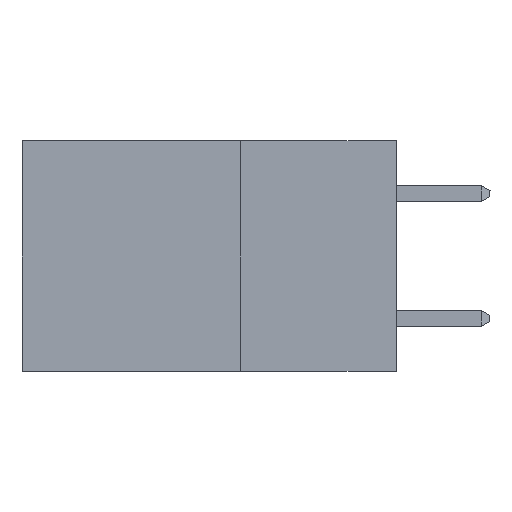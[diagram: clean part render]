
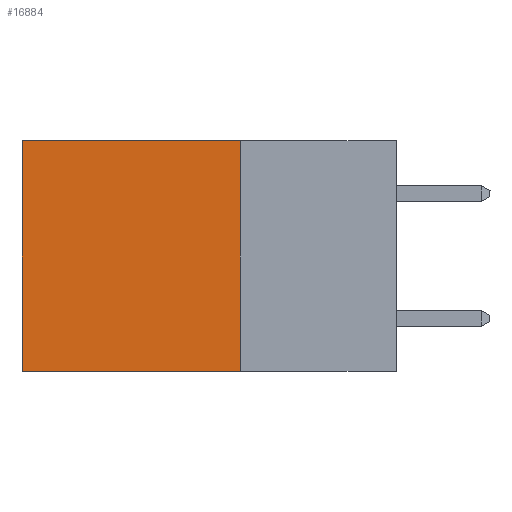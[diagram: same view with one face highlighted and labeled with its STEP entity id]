
A CAD part, left-side view. The second image highlights one B-rep face of the part: STEP entity #16884.
In plain terms, the highlighted planar face has unit normal (-1, 0, 0).
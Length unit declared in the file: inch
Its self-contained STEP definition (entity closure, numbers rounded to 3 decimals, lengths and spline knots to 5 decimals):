
#1252 = EDGE_CURVE ( 'NONE', #13404, #5144, #9243, .T. ) ;
#2403 = PLANE ( 'NONE',  #3668 ) ;
#2669 = ORIENTED_EDGE ( 'NONE', *, *, #17955, .T. ) ;
#3668 = AXIS2_PLACEMENT_3D ( 'NONE', #14720, #4499, #18843 ) ;
#4201 = CARTESIAN_POINT ( 'NONE',  ( 0.2615, 0.25, -0.37 ) ) ;
#4499 = DIRECTION ( 'NONE',  ( 1., 0., 0. ) ) ;
#4876 = EDGE_CURVE ( 'NONE', #19270, #9425, #12886, .T. ) ;
#5144 = VERTEX_POINT ( 'NONE', #4201 ) ;
#9243 = LINE ( 'NONE', #21538, #14675 ) ;
#9425 = VERTEX_POINT ( 'NONE', #18350 ) ;
#9893 = ORIENTED_EDGE ( 'NONE', *, *, #14242, .F. ) ;
#10083 = ORIENTED_EDGE ( 'NONE', *, *, #1252, .F. ) ;
#11781 = CARTESIAN_POINT ( 'NONE',  ( 0.2615, 0.6, -0.37 ) ) ;
#12010 = LINE ( 'NONE', #18688, #17463 ) ;
#12070 = DIRECTION ( 'NONE',  ( 0., 0., -1. ) ) ;
#12886 = LINE ( 'NONE', #11781, #22431 ) ;
#13404 = VERTEX_POINT ( 'NONE', #16873 ) ;
#14242 = EDGE_CURVE ( 'NONE', #5144, #9425, #12010, .T. ) ;
#14675 = VECTOR ( 'NONE', #21311, 39.37008 ) ;
#14682 = EDGE_LOOP ( 'NONE', ( #23050, #9893, #10083, #2669 ) ) ;
#14720 = CARTESIAN_POINT ( 'NONE',  ( 0.2615, 0.25, -0.37 ) ) ;
#15757 = VECTOR ( 'NONE', #22802, 39.37008 ) ;
#16873 = CARTESIAN_POINT ( 'NONE',  ( 0.2615, 0.25, 0. ) ) ;
#16884 = ADVANCED_FACE ( 'NONE', ( #23760 ), #2403, .F. ) ;
#17463 = VECTOR ( 'NONE', #24718, 39.37008 ) ;
#17955 = EDGE_CURVE ( 'NONE', #13404, #19270, #21166, .T. ) ;
#18350 = CARTESIAN_POINT ( 'NONE',  ( 0.2615, 0.6, -0.37 ) ) ;
#18688 = CARTESIAN_POINT ( 'NONE',  ( 0.2615, 0.25, -0.37 ) ) ;
#18843 = DIRECTION ( 'NONE',  ( 0., 0., -1. ) ) ;
#19270 = VERTEX_POINT ( 'NONE', #20891 ) ;
#20772 = CARTESIAN_POINT ( 'NONE',  ( 0.2615, 0.25, 0. ) ) ;
#20891 = CARTESIAN_POINT ( 'NONE',  ( 0.2615, 0.6, 0. ) ) ;
#21166 = LINE ( 'NONE', #20772, #15757 ) ;
#21311 = DIRECTION ( 'NONE',  ( 0., 0., -1. ) ) ;
#21538 = CARTESIAN_POINT ( 'NONE',  ( 0.2615, 0.25, -0.37 ) ) ;
#22431 = VECTOR ( 'NONE', #12070, 39.37008 ) ;
#22802 = DIRECTION ( 'NONE',  ( 0., 1., 0. ) ) ;
#23050 = ORIENTED_EDGE ( 'NONE', *, *, #4876, .T. ) ;
#23760 = FACE_OUTER_BOUND ( 'NONE', #14682, .T. ) ;
#24718 = DIRECTION ( 'NONE',  ( 0., 1., 0. ) ) ;
